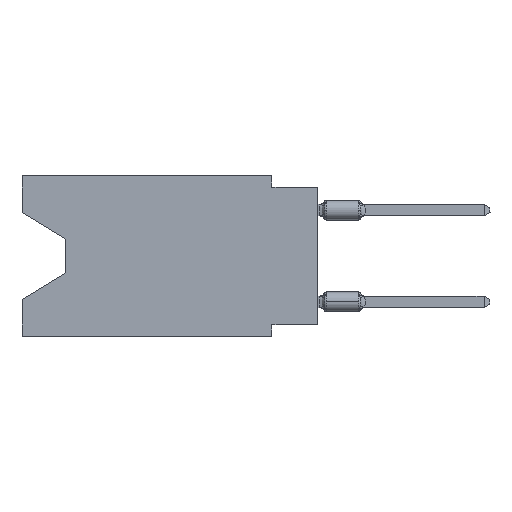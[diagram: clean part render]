
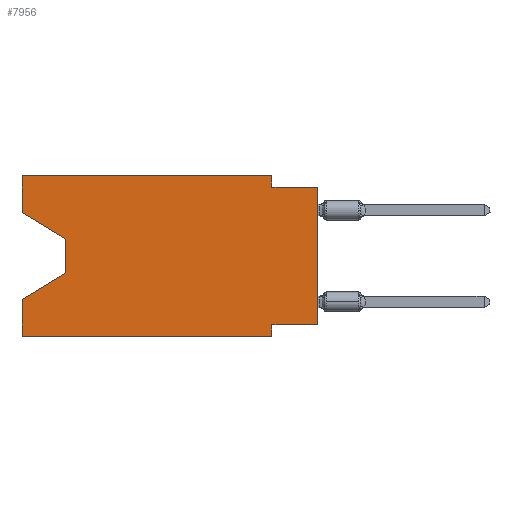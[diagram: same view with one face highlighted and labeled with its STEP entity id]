
A CAD part, left-side view. The second image highlights one B-rep face of the part: STEP entity #7956.
In plain terms, the highlighted planar face has unit normal (-1, 0, 0).
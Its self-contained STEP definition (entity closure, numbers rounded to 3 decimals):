
#39 = CARTESIAN_POINT ( 'NONE',  ( 0., 16.383, 0. ) ) ;
#810 = LINE ( 'NONE', #26684, #33569 ) ;
#835 = DIRECTION ( 'NONE',  ( 0., 0., 1. ) ) ;
#1016 = CARTESIAN_POINT ( 'NONE',  ( 0., 16.383, 0. ) ) ;
#1216 = CARTESIAN_POINT ( 'NONE',  ( 0., 16.383, -8.89 ) ) ;
#1382 = EDGE_CURVE ( 'NONE', #6378, #33471, #23991, .T. ) ;
#1418 = CARTESIAN_POINT ( 'NONE',  ( 0., 16.383, -2.038 ) ) ;
#1482 = CARTESIAN_POINT ( 'NONE',  ( 0., 16.383, -2.038 ) ) ;
#1850 = CARTESIAN_POINT ( 'NONE',  ( 0., 2.54, -0.635 ) ) ;
#2086 = AXIS2_PLACEMENT_3D ( 'NONE', #11611, #6355, #29825 ) ;
#2128 = EDGE_CURVE ( 'NONE', #17706, #11083, #23357, .T. ) ;
#2433 = VERTEX_POINT ( 'NONE', #5286 ) ;
#2693 = LINE ( 'NONE', #13061, #29815 ) ;
#2716 = ORIENTED_EDGE ( 'NONE', *, *, #32666, .T. ) ;
#3499 = CARTESIAN_POINT ( 'NONE',  ( 0., 13.97, -3.505 ) ) ;
#3886 = LINE ( 'NONE', #16616, #15142 ) ;
#3996 = CARTESIAN_POINT ( 'NONE',  ( 0., 0., -8.255 ) ) ;
#4984 = DIRECTION ( 'NONE',  ( 0., 0., 1. ) ) ;
#5286 = CARTESIAN_POINT ( 'NONE',  ( 0., 0., -0.635 ) ) ;
#5503 = VERTEX_POINT ( 'NONE', #3996 ) ;
#5699 = VERTEX_POINT ( 'NONE', #31483 ) ;
#6355 = DIRECTION ( 'NONE',  ( 1., 0., 0. ) ) ;
#6378 = VERTEX_POINT ( 'NONE', #1482 ) ;
#6537 = VECTOR ( 'NONE', #835, 1000. ) ;
#6562 = VECTOR ( 'NONE', #4984, 1000. ) ;
#6783 = DIRECTION ( 'NONE',  ( 0., -1., 0. ) ) ;
#7956 = ADVANCED_FACE ( 'NONE', ( #22168 ), #27254, .F. ) ;
#9130 = DIRECTION ( 'NONE',  ( 0., 0.855, -0.519 ) ) ;
#9394 = EDGE_CURVE ( 'NONE', #33471, #11180, #23671, .T. ) ;
#9569 = ORIENTED_EDGE ( 'NONE', *, *, #27922, .F. ) ;
#10863 = VECTOR ( 'NONE', #18417, 1000. ) ;
#11083 = VERTEX_POINT ( 'NONE', #32136 ) ;
#11180 = VERTEX_POINT ( 'NONE', #31403 ) ;
#11417 = ORIENTED_EDGE ( 'NONE', *, *, #14251, .F. ) ;
#11611 = CARTESIAN_POINT ( 'NONE',  ( 0., 16.383, 0. ) ) ;
#11801 = DIRECTION ( 'NONE',  ( 0., -0.855, -0.519 ) ) ;
#12826 = CARTESIAN_POINT ( 'NONE',  ( 0., 2.54, -8.89 ) ) ;
#13061 = CARTESIAN_POINT ( 'NONE',  ( 0., 13.97, -5.385 ) ) ;
#13293 = EDGE_CURVE ( 'NONE', #27012, #2433, #21951, .T. ) ;
#13335 = CARTESIAN_POINT ( 'NONE',  ( 0., 2.54, -8.255 ) ) ;
#13594 = DIRECTION ( 'NONE',  ( 0., 0., 1. ) ) ;
#14251 = EDGE_CURVE ( 'NONE', #14439, #30886, #33393, .T. ) ;
#14386 = VECTOR ( 'NONE', #21075, 1000. ) ;
#14439 = VERTEX_POINT ( 'NONE', #13335 ) ;
#14452 = CARTESIAN_POINT ( 'NONE',  ( 0., 0., -0.635 ) ) ;
#15142 = VECTOR ( 'NONE', #26993, 1000. ) ;
#15513 = ORIENTED_EDGE ( 'NONE', *, *, #1382, .F. ) ;
#15682 = EDGE_CURVE ( 'NONE', #5503, #14439, #21882, .T. ) ;
#15950 = ORIENTED_EDGE ( 'NONE', *, *, #9394, .F. ) ;
#16616 = CARTESIAN_POINT ( 'NONE',  ( 0., 16.383, -8.89 ) ) ;
#17706 = VERTEX_POINT ( 'NONE', #1216 ) ;
#18417 = DIRECTION ( 'NONE',  ( 0., -1., 0. ) ) ;
#18681 = CARTESIAN_POINT ( 'NONE',  ( 0., 13.97, -3.505 ) ) ;
#21075 = DIRECTION ( 'NONE',  ( 0., 0., -1. ) ) ;
#21304 = EDGE_CURVE ( 'NONE', #30464, #5699, #28372, .T. ) ;
#21416 = CARTESIAN_POINT ( 'NONE',  ( 0., 2.54, -8.89 ) ) ;
#21727 = DIRECTION ( 'NONE',  ( 0., 1., 0. ) ) ;
#21882 = LINE ( 'NONE', #24918, #32546 ) ;
#21951 = LINE ( 'NONE', #14452, #33555 ) ;
#22168 = FACE_OUTER_BOUND ( 'NONE', #24281, .T. ) ;
#23357 = LINE ( 'NONE', #39, #6562 ) ;
#23671 = LINE ( 'NONE', #28949, #10863 ) ;
#23719 = DIRECTION ( 'NONE',  ( 0., 0., -1. ) ) ;
#23991 = LINE ( 'NONE', #1016, #6537 ) ;
#24281 = EDGE_LOOP ( 'NONE', ( #32108, #28886, #28815, #29307, #2716, #11417, #26733, #25149, #27576, #9569, #15950, #15513 ) ) ;
#24715 = LINE ( 'NONE', #1418, #28532 ) ;
#24879 = EDGE_CURVE ( 'NONE', #5503, #2433, #810, .T. ) ;
#24918 = CARTESIAN_POINT ( 'NONE',  ( 0., 0., -8.255 ) ) ;
#25149 = ORIENTED_EDGE ( 'NONE', *, *, #24879, .T. ) ;
#25742 = DIRECTION ( 'NONE',  ( 0., 0., -1. ) ) ;
#26065 = CARTESIAN_POINT ( 'NONE',  ( 0., 16.383, 0. ) ) ;
#26684 = CARTESIAN_POINT ( 'NONE',  ( 0., 0., 0. ) ) ;
#26733 = ORIENTED_EDGE ( 'NONE', *, *, #15682, .F. ) ;
#26993 = DIRECTION ( 'NONE',  ( 0., -1., 0. ) ) ;
#27012 = VERTEX_POINT ( 'NONE', #1850 ) ;
#27254 = PLANE ( 'NONE',  #2086 ) ;
#27576 = ORIENTED_EDGE ( 'NONE', *, *, #13293, .F. ) ;
#27922 = EDGE_CURVE ( 'NONE', #11180, #27012, #33587, .T. ) ;
#28057 = VECTOR ( 'NONE', #23719, 1000. ) ;
#28372 = LINE ( 'NONE', #18681, #14386 ) ;
#28532 = VECTOR ( 'NONE', #11801, 1000. ) ;
#28651 = CARTESIAN_POINT ( 'NONE',  ( 0., 2.54, 0. ) ) ;
#28815 = ORIENTED_EDGE ( 'NONE', *, *, #32612, .T. ) ;
#28886 = ORIENTED_EDGE ( 'NONE', *, *, #21304, .T. ) ;
#28949 = CARTESIAN_POINT ( 'NONE',  ( 0., 16.383, 0. ) ) ;
#29307 = ORIENTED_EDGE ( 'NONE', *, *, #2128, .F. ) ;
#29815 = VECTOR ( 'NONE', #9130, 1000. ) ;
#29825 = DIRECTION ( 'NONE',  ( 0., 0., -1. ) ) ;
#30464 = VERTEX_POINT ( 'NONE', #3499 ) ;
#30886 = VERTEX_POINT ( 'NONE', #21416 ) ;
#31403 = CARTESIAN_POINT ( 'NONE',  ( 0., 2.54, 0. ) ) ;
#31483 = CARTESIAN_POINT ( 'NONE',  ( 0., 13.97, -5.385 ) ) ;
#32108 = ORIENTED_EDGE ( 'NONE', *, *, #33177, .T. ) ;
#32136 = CARTESIAN_POINT ( 'NONE',  ( 0., 16.383, -6.852 ) ) ;
#32546 = VECTOR ( 'NONE', #21727, 1000. ) ;
#32612 = EDGE_CURVE ( 'NONE', #5699, #11083, #2693, .T. ) ;
#32666 = EDGE_CURVE ( 'NONE', #17706, #30886, #3886, .T. ) ;
#33177 = EDGE_CURVE ( 'NONE', #6378, #30464, #24715, .T. ) ;
#33393 = LINE ( 'NONE', #12826, #33615 ) ;
#33471 = VERTEX_POINT ( 'NONE', #26065 ) ;
#33555 = VECTOR ( 'NONE', #6783, 1000. ) ;
#33569 = VECTOR ( 'NONE', #13594, 1000. ) ;
#33587 = LINE ( 'NONE', #28651, #28057 ) ;
#33615 = VECTOR ( 'NONE', #25742, 1000. ) ;
